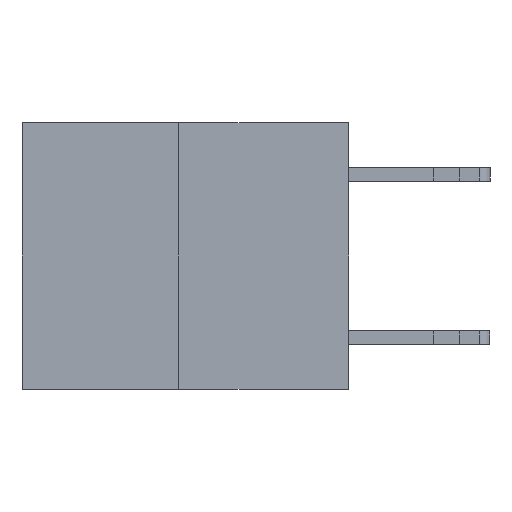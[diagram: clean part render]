
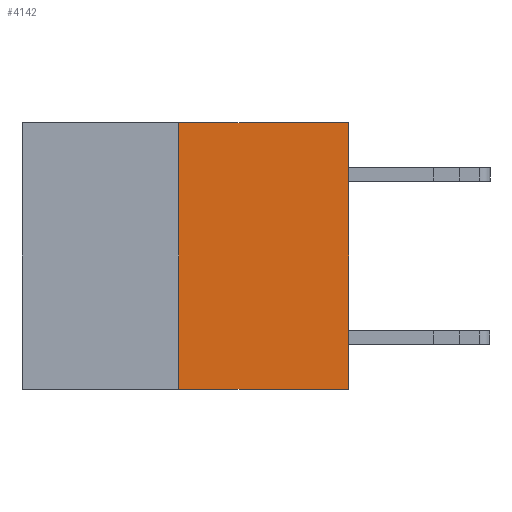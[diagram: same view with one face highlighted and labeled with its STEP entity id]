
A CAD part, left-side view. The second image highlights one B-rep face of the part: STEP entity #4142.
In plain terms, the highlighted planar face has unit normal (-1, 0, 0).
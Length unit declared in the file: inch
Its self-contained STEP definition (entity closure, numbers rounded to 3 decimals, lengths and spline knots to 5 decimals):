
#402 = CARTESIAN_POINT ( 'NONE',  ( 0., 0.312, 0. ) ) ;
#895 = EDGE_CURVE ( 'NONE', #13089, #4377, #10465, .T. ) ;
#1361 = DIRECTION ( 'NONE',  ( 0., 0., 1. ) ) ;
#2888 = ORIENTED_EDGE ( 'NONE', *, *, #10633, .F. ) ;
#2995 = AXIS2_PLACEMENT_3D ( 'NONE', #4225, #4371, #5383 ) ;
#3234 = VECTOR ( 'NONE', #5912, 39.37008 ) ;
#4142 = ADVANCED_FACE ( 'NONE', ( #4764 ), #9814, .F. ) ;
#4225 = CARTESIAN_POINT ( 'NONE',  ( 0., 0.6, 0. ) ) ;
#4371 = DIRECTION ( 'NONE',  ( 1., 0., 0. ) ) ;
#4377 = VERTEX_POINT ( 'NONE', #6560 ) ;
#4693 = CARTESIAN_POINT ( 'NONE',  ( 0., 0.312, -0.49 ) ) ;
#4764 = FACE_OUTER_BOUND ( 'NONE', #11707, .T. ) ;
#5383 = DIRECTION ( 'NONE',  ( 0., 0., -1. ) ) ;
#5912 = DIRECTION ( 'NONE',  ( 0., -1., 0. ) ) ;
#6072 = EDGE_CURVE ( 'NONE', #13089, #11710, #7871, .T. ) ;
#6257 = EDGE_CURVE ( 'NONE', #4377, #7440, #14226, .T. ) ;
#6345 = VECTOR ( 'NONE', #12690, 39.37008 ) ;
#6560 = CARTESIAN_POINT ( 'NONE',  ( 0., 0., -0.49 ) ) ;
#7440 = VERTEX_POINT ( 'NONE', #13539 ) ;
#7573 = LINE ( 'NONE', #10401, #3234 ) ;
#7618 = CARTESIAN_POINT ( 'NONE',  ( 0., 0., 0. ) ) ;
#7871 = LINE ( 'NONE', #13516, #11642 ) ;
#8014 = ORIENTED_EDGE ( 'NONE', *, *, #895, .T. ) ;
#8278 = ORIENTED_EDGE ( 'NONE', *, *, #6257, .T. ) ;
#8739 = ORIENTED_EDGE ( 'NONE', *, *, #6072, .F. ) ;
#9814 = PLANE ( 'NONE',  #2995 ) ;
#10401 = CARTESIAN_POINT ( 'NONE',  ( 0., 0.6, 0. ) ) ;
#10465 = LINE ( 'NONE', #11701, #6345 ) ;
#10633 = EDGE_CURVE ( 'NONE', #11710, #7440, #7573, .T. ) ;
#11282 = VECTOR ( 'NONE', #13289, 39.37008 ) ;
#11642 = VECTOR ( 'NONE', #1361, 39.37008 ) ;
#11701 = CARTESIAN_POINT ( 'NONE',  ( 0., 0.6, -0.49 ) ) ;
#11707 = EDGE_LOOP ( 'NONE', ( #8739, #8014, #8278, #2888 ) ) ;
#11710 = VERTEX_POINT ( 'NONE', #402 ) ;
#12690 = DIRECTION ( 'NONE',  ( 0., -1., 0. ) ) ;
#13089 = VERTEX_POINT ( 'NONE', #4693 ) ;
#13289 = DIRECTION ( 'NONE',  ( 0., 0., 1. ) ) ;
#13516 = CARTESIAN_POINT ( 'NONE',  ( 0., 0.312, -0.49 ) ) ;
#13539 = CARTESIAN_POINT ( 'NONE',  ( 0., 0., 0. ) ) ;
#14226 = LINE ( 'NONE', #7618, #11282 ) ;
